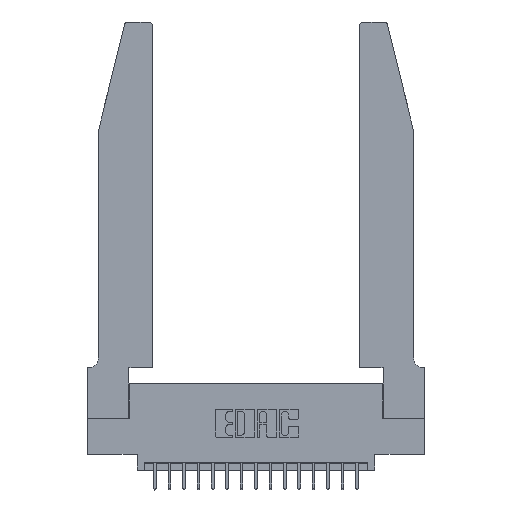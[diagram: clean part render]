
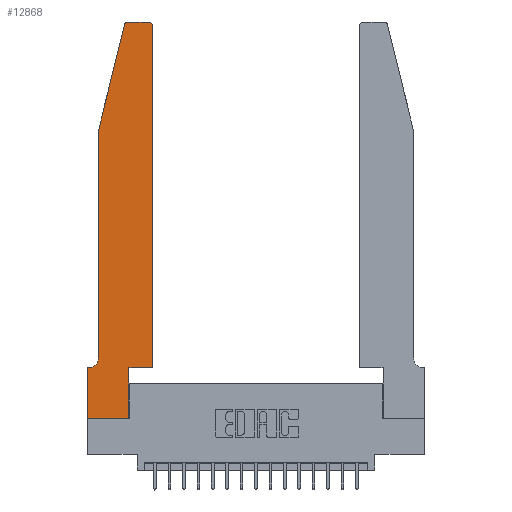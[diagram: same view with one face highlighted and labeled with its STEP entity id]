
A CAD part, top view. The second image highlights one B-rep face of the part: STEP entity #12868.
In plain terms, the highlighted planar face has unit normal (0, 0, 1).
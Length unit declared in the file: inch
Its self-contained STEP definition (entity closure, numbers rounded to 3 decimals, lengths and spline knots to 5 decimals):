
#201 = ORIENTED_EDGE ( 'NONE', *, *, #18330, .T. ) ;
#233 = DIRECTION ( 'NONE',  ( 1., 0., 0. ) ) ;
#880 = DIRECTION ( 'NONE',  ( 0., -1., 0. ) ) ;
#883 = VERTEX_POINT ( 'NONE', #18059 ) ;
#1654 = DIRECTION ( 'NONE',  ( 0., -1., 0. ) ) ;
#1832 = DIRECTION ( 'NONE',  ( 1., 0., 0. ) ) ;
#1919 = ORIENTED_EDGE ( 'NONE', *, *, #9227, .T. ) ;
#2741 = DIRECTION ( 'NONE',  ( 0., 1., 0. ) ) ;
#2794 = DIRECTION ( 'NONE',  ( -1., 0., 0. ) ) ;
#3415 = VERTEX_POINT ( 'NONE', #9733 ) ;
#3474 = VERTEX_POINT ( 'NONE', #13302 ) ;
#3706 = AXIS2_PLACEMENT_3D ( 'NONE', #9719, #17583, #8180 ) ;
#4362 = ORIENTED_EDGE ( 'NONE', *, *, #11963, .T. ) ;
#4409 = ORIENTED_EDGE ( 'NONE', *, *, #9998, .T. ) ;
#4466 = DIRECTION ( 'NONE',  ( 0., 0., -1. ) ) ;
#4478 = FACE_OUTER_BOUND ( 'NONE', #7054, .T. ) ;
#4538 = CARTESIAN_POINT ( 'NONE',  ( 0.25487, 2.72718, 0.37 ) ) ;
#4616 = LINE ( 'NONE', #16054, #6291 ) ;
#4625 = ORIENTED_EDGE ( 'NONE', *, *, #13597, .T. ) ;
#4842 = ORIENTED_EDGE ( 'NONE', *, *, #16039, .T. ) ;
#4967 = CARTESIAN_POINT ( 'NONE',  ( 0., 0.35, 0.37 ) ) ;
#5171 = VERTEX_POINT ( 'NONE', #16072 ) ;
#5312 = VERTEX_POINT ( 'NONE', #17679 ) ;
#5348 = ORIENTED_EDGE ( 'NONE', *, *, #15810, .T. ) ;
#5476 = AXIS2_PLACEMENT_3D ( 'NONE', #12048, #4466, #2794 ) ;
#5801 = LINE ( 'NONE', #10538, #16455 ) ;
#5824 = CARTESIAN_POINT ( 'NONE',  ( 0.0755, 2., 0.37 ) ) ;
#5862 = VERTEX_POINT ( 'NONE', #11098 ) ;
#5888 = ORIENTED_EDGE ( 'NONE', *, *, #14469, .T. ) ;
#6058 = EDGE_CURVE ( 'NONE', #3415, #8400, #4616, .T. ) ;
#6085 = CARTESIAN_POINT ( 'NONE',  ( 0.284, 2.72, 0.37 ) ) ;
#6291 = VECTOR ( 'NONE', #1832, 39.37008 ) ;
#6386 = DIRECTION ( 'NONE',  ( 1., 0., 0. ) ) ;
#6805 = DIRECTION ( 'NONE',  ( -1., 0., 0. ) ) ;
#7054 = EDGE_LOOP ( 'NONE', ( #4409, #1919, #4362, #201, #5888, #4625, #5348, #16145, #20111, #16380, #4842, #8342 ) ) ;
#7947 = DIRECTION ( 'NONE',  ( 0., 0., 1. ) ) ;
#8143 = LINE ( 'NONE', #9887, #16242 ) ;
#8176 = VECTOR ( 'NONE', #18246, 39.37008 ) ;
#8180 = DIRECTION ( 'NONE',  ( 1., 0., 0. ) ) ;
#8257 = CARTESIAN_POINT ( 'NONE',  ( 0.4505, 2.72, 0.37 ) ) ;
#8342 = ORIENTED_EDGE ( 'NONE', *, *, #19483, .T. ) ;
#8358 = CARTESIAN_POINT ( 'NONE',  ( 0.2605, 2.75, 0.37 ) ) ;
#8391 = EDGE_CURVE ( 'NONE', #883, #5862, #8143, .T. ) ;
#8400 = VERTEX_POINT ( 'NONE', #14438 ) ;
#9227 = EDGE_CURVE ( 'NONE', #5312, #9250, #19917, .T. ) ;
#9250 = VERTEX_POINT ( 'NONE', #4538 ) ;
#9719 = CARTESIAN_POINT ( 'NONE',  ( 0.4205, 2.72, 0.37 ) ) ;
#9733 = CARTESIAN_POINT ( 'NONE',  ( 0., 0., 0.37 ) ) ;
#9885 = CIRCLE ( 'NONE', #3706, 0.03 ) ;
#9887 = CARTESIAN_POINT ( 'NONE',  ( 0.4505, 0.35, 0.37 ) ) ;
#9998 = EDGE_CURVE ( 'NONE', #19155, #5312, #10394, .T. ) ;
#10146 = LINE ( 'NONE', #5824, #15333 ) ;
#10394 = LINE ( 'NONE', #8358, #16929 ) ;
#10538 = CARTESIAN_POINT ( 'NONE',  ( 0.0755, 2., 0.37 ) ) ;
#10577 = CARTESIAN_POINT ( 'NONE',  ( 0.4505, 0.35, 0.37 ) ) ;
#11096 = VECTOR ( 'NONE', #2741, 39.37008 ) ;
#11098 = CARTESIAN_POINT ( 'NONE',  ( 0.4505, 0.35, 0.37 ) ) ;
#11210 = VERTEX_POINT ( 'NONE', #19426 ) ;
#11371 = LINE ( 'NONE', #17695, #19641 ) ;
#11507 = CARTESIAN_POINT ( 'NONE',  ( 0.4205, 2.75, 0.37 ) ) ;
#11963 = EDGE_CURVE ( 'NONE', #9250, #19004, #10146, .T. ) ;
#12048 = CARTESIAN_POINT ( 'NONE',  ( 0.0055, 0.42, 0.37 ) ) ;
#12067 = VECTOR ( 'NONE', #1654, 39.37008 ) ;
#12615 = LINE ( 'NONE', #10577, #11096 ) ;
#12868 = ADVANCED_FACE ( 'NONE', ( #4478 ), #19138, .T. ) ;
#13015 = CIRCLE ( 'NONE', #5476, 0.07 ) ;
#13302 = CARTESIAN_POINT ( 'NONE',  ( 0.0755, 0.42, 0.37 ) ) ;
#13597 = EDGE_CURVE ( 'NONE', #5171, #11210, #11371, .T. ) ;
#14048 = AXIS2_PLACEMENT_3D ( 'NONE', #4967, #7947, #15612 ) ;
#14316 = CARTESIAN_POINT ( 'NONE',  ( 0.0755, 2., 0.37 ) ) ;
#14438 = CARTESIAN_POINT ( 'NONE',  ( 0.2865, 0., 0.37 ) ) ;
#14469 = EDGE_CURVE ( 'NONE', #3474, #5171, #13015, .T. ) ;
#15020 = LINE ( 'NONE', #15227, #8176 ) ;
#15227 = CARTESIAN_POINT ( 'NONE',  ( 0.2865, 0.35, 0.37 ) ) ;
#15333 = VECTOR ( 'NONE', #17911, 39.37008 ) ;
#15612 = DIRECTION ( 'NONE',  ( 1., 0., 0. ) ) ;
#15646 = VERTEX_POINT ( 'NONE', #8257 ) ;
#15787 = CARTESIAN_POINT ( 'NONE',  ( 0., 0., 0.37 ) ) ;
#15810 = EDGE_CURVE ( 'NONE', #11210, #3415, #17319, .T. ) ;
#16039 = EDGE_CURVE ( 'NONE', #5862, #15646, #12615, .T. ) ;
#16054 = CARTESIAN_POINT ( 'NONE',  ( 0., 0., 0.37 ) ) ;
#16072 = CARTESIAN_POINT ( 'NONE',  ( 0.0055, 0.35, 0.37 ) ) ;
#16145 = ORIENTED_EDGE ( 'NONE', *, *, #6058, .T. ) ;
#16242 = VECTOR ( 'NONE', #6386, 39.37008 ) ;
#16268 = AXIS2_PLACEMENT_3D ( 'NONE', #6085, #17322, #233 ) ;
#16380 = ORIENTED_EDGE ( 'NONE', *, *, #8391, .T. ) ;
#16455 = VECTOR ( 'NONE', #880, 39.37008 ) ;
#16588 = EDGE_CURVE ( 'NONE', #8400, #883, #15020, .T. ) ;
#16929 = VECTOR ( 'NONE', #6805, 39.37008 ) ;
#17319 = LINE ( 'NONE', #15787, #12067 ) ;
#17322 = DIRECTION ( 'NONE',  ( 0., 0., 1. ) ) ;
#17583 = DIRECTION ( 'NONE',  ( 0., 0., 1. ) ) ;
#17679 = CARTESIAN_POINT ( 'NONE',  ( 0.284, 2.75, 0.37 ) ) ;
#17695 = CARTESIAN_POINT ( 'NONE',  ( 0.0755, 0.35, 0.37 ) ) ;
#17911 = DIRECTION ( 'NONE',  ( -0.239, -0.971, 0. ) ) ;
#18059 = CARTESIAN_POINT ( 'NONE',  ( 0.2865, 0.35, 0.37 ) ) ;
#18246 = DIRECTION ( 'NONE',  ( 0., 1., 0. ) ) ;
#18330 = EDGE_CURVE ( 'NONE', #19004, #3474, #5801, .T. ) ;
#19004 = VERTEX_POINT ( 'NONE', #14316 ) ;
#19138 = PLANE ( 'NONE',  #14048 ) ;
#19155 = VERTEX_POINT ( 'NONE', #11507 ) ;
#19373 = DIRECTION ( 'NONE',  ( -1., 0., 0. ) ) ;
#19426 = CARTESIAN_POINT ( 'NONE',  ( 0., 0.35, 0.37 ) ) ;
#19483 = EDGE_CURVE ( 'NONE', #15646, #19155, #9885, .T. ) ;
#19641 = VECTOR ( 'NONE', #19373, 39.37008 ) ;
#19917 = CIRCLE ( 'NONE', #16268, 0.03 ) ;
#20111 = ORIENTED_EDGE ( 'NONE', *, *, #16588, .T. ) ;
